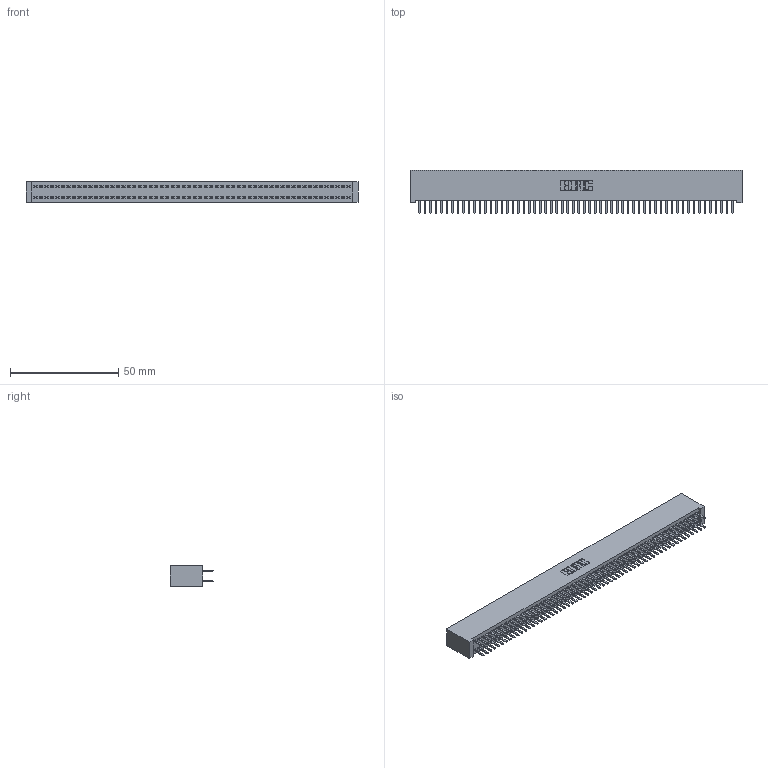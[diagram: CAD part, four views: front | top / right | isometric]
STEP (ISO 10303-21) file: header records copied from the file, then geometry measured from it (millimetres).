
FILE_DESCRIPTION (( 'STEP AP203' ), '1' );
FILE_NAME ('342-116-520-201.STEP', '2019-10-04T21:59:07', ( '' ), ( '' ), 'SwSTEP 2.0', 'SolidWorks 2016', '' );
FILE_SCHEMA (( 'CONFIG_CONTROL_DESIGN' ));
Length unit declared in the file: inch
Products named in the file (3): 342 Part_Lugless; 345-292-001_345-293-120; 342-116-520-201
Assembly tree (117 placements, depth 2):
  342-116-520-201
    342 Part_Lugless
    345-292-001_345-293-120  x116
Bounding box: 153.57 x 20.02 x 9.4 mm (x, y, z)
Volume: 14262.3 mm3; surface area: 23935.7 mm2
Topology: 117 solids, 117 shells, 6598 faces, 19183 edges, 12478 vertices
Faces by surface type: plane 4470, cylinder 2128
Entity records: 34949 total; most frequent: CARTESIAN_POINT 5782, ORIENTED_EDGE 5706, DIRECTION 4893, EDGE_CURVE 2853, LINE 2729, VECTOR 2729, VERTEX_POINT 1898, AXIS2_PLACEMENT_3D 1082
